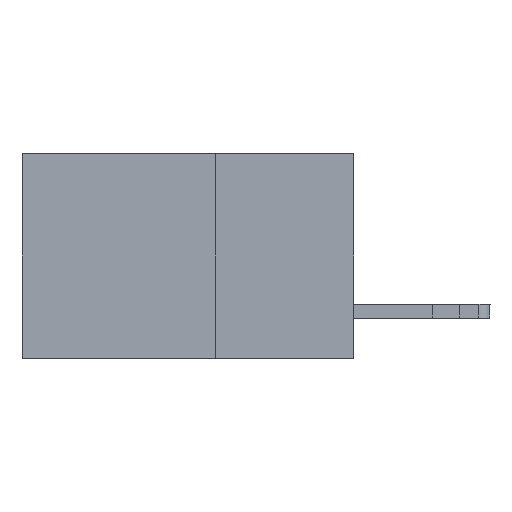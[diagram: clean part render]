
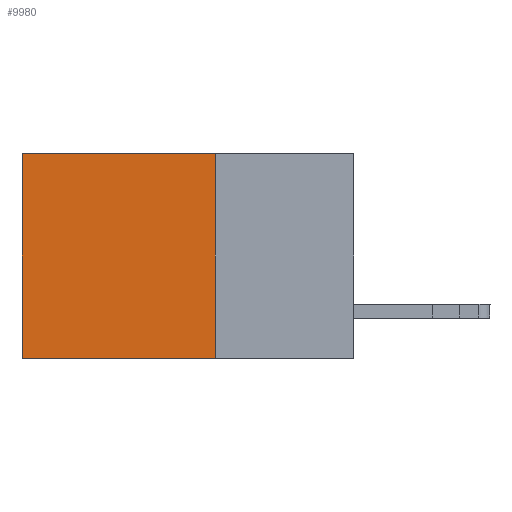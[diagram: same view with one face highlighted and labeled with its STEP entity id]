
A CAD part, left-side view. The second image highlights one B-rep face of the part: STEP entity #9980.
In plain terms, the highlighted planar face has unit normal (-1, 0, 0).
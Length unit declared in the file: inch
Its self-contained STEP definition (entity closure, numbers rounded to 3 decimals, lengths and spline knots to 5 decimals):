
#244 = DIRECTION ( 'NONE',  ( 0., 1., 0. ) ) ;
#374 = CARTESIAN_POINT ( 'NONE',  ( 0.2875, 0.6, 0. ) ) ;
#860 = VECTOR ( 'NONE', #2863, 39.37008 ) ;
#1247 = VERTEX_POINT ( 'NONE', #10878 ) ;
#1719 = ORIENTED_EDGE ( 'NONE', *, *, #11651, .T. ) ;
#2136 = LINE ( 'NONE', #5260, #8328 ) ;
#2368 = CARTESIAN_POINT ( 'NONE',  ( 0.2875, 0.6, -0.37 ) ) ;
#2863 = DIRECTION ( 'NONE',  ( 0., 0., -1. ) ) ;
#3074 = VERTEX_POINT ( 'NONE', #2368 ) ;
#3090 = DIRECTION ( 'NONE',  ( 0., 1., 0. ) ) ;
#3254 = FACE_OUTER_BOUND ( 'NONE', #12292, .T. ) ;
#3392 = EDGE_CURVE ( 'NONE', #11678, #14179, #8600, .T. ) ;
#4543 = LINE ( 'NONE', #9183, #11099 ) ;
#5017 = ORIENTED_EDGE ( 'NONE', *, *, #3392, .F. ) ;
#5260 = CARTESIAN_POINT ( 'NONE',  ( 0.2875, 0.25, -0.37 ) ) ;
#5894 = DIRECTION ( 'NONE',  ( 1., 0., 0. ) ) ;
#6477 = VECTOR ( 'NONE', #11488, 39.37008 ) ;
#8014 = LINE ( 'NONE', #374, #860 ) ;
#8171 = DIRECTION ( 'NONE',  ( 0., 0., -1. ) ) ;
#8328 = VECTOR ( 'NONE', #244, 39.37008 ) ;
#8600 = LINE ( 'NONE', #12676, #6477 ) ;
#9183 = CARTESIAN_POINT ( 'NONE',  ( 0.2875, 0.25, 0. ) ) ;
#9980 = ADVANCED_FACE ( 'NONE', ( #3254 ), #15727, .F. ) ;
#10161 = CARTESIAN_POINT ( 'NONE',  ( 0.2875, 0.25, 0. ) ) ;
#10878 = CARTESIAN_POINT ( 'NONE',  ( 0.2875, 0.6, 0. ) ) ;
#11099 = VECTOR ( 'NONE', #3090, 39.37008 ) ;
#11488 = DIRECTION ( 'NONE',  ( 0., 0., -1. ) ) ;
#11651 = EDGE_CURVE ( 'NONE', #1247, #3074, #8014, .T. ) ;
#11678 = VERTEX_POINT ( 'NONE', #10161 ) ;
#12041 = AXIS2_PLACEMENT_3D ( 'NONE', #13326, #5894, #8171 ) ;
#12292 = EDGE_LOOP ( 'NONE', ( #1719, #15434, #5017, #15762 ) ) ;
#12676 = CARTESIAN_POINT ( 'NONE',  ( 0.2875, 0.25, 0. ) ) ;
#13193 = CARTESIAN_POINT ( 'NONE',  ( 0.2875, 0.25, -0.37 ) ) ;
#13326 = CARTESIAN_POINT ( 'NONE',  ( 0.2875, 0.25, 0. ) ) ;
#13875 = EDGE_CURVE ( 'NONE', #14179, #3074, #2136, .T. ) ;
#14179 = VERTEX_POINT ( 'NONE', #13193 ) ;
#15434 = ORIENTED_EDGE ( 'NONE', *, *, #13875, .F. ) ;
#15637 = EDGE_CURVE ( 'NONE', #11678, #1247, #4543, .T. ) ;
#15727 = PLANE ( 'NONE',  #12041 ) ;
#15762 = ORIENTED_EDGE ( 'NONE', *, *, #15637, .T. ) ;
